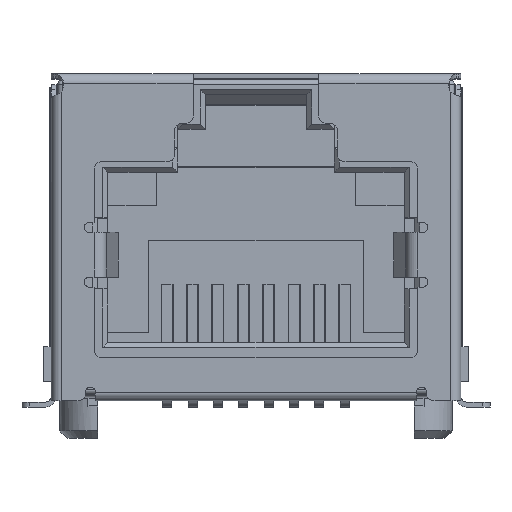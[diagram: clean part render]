
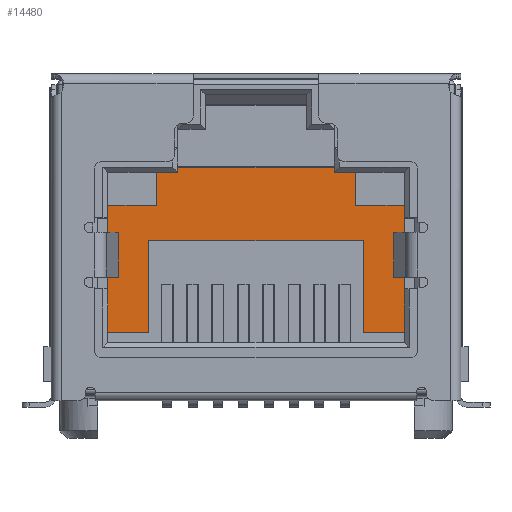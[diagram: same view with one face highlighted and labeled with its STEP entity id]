
A CAD part, top view. The second image highlights one B-rep face of the part: STEP entity #14480.
In plain terms, the highlighted planar face has unit normal (0, 0, 1).
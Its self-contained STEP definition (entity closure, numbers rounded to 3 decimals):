
#63 = ORIENTED_EDGE ( 'NONE', *, *, #17786, .T. ) ;
#538 = LINE ( 'NONE', #16832, #18644 ) ;
#540 = CARTESIAN_POINT ( 'NONE',  ( 13.93, 2.65, -12. ) ) ;
#629 = EDGE_CURVE ( 'NONE', #1205, #18476, #13843, .T. ) ;
#880 = DIRECTION ( 'NONE',  ( -1., 0., 0. ) ) ;
#1205 = VERTEX_POINT ( 'NONE', #23132 ) ;
#1334 = VECTOR ( 'NONE', #18363, 1000. ) ;
#1976 = ORIENTED_EDGE ( 'NONE', *, *, #15438, .T. ) ;
#2643 = VERTEX_POINT ( 'NONE', #22831 ) ;
#3051 = CARTESIAN_POINT ( 'NONE',  ( 3.675, 2.65, -12. ) ) ;
#3092 = LINE ( 'NONE', #10632, #17224 ) ;
#3462 = VECTOR ( 'NONE', #11119, 1000. ) ;
#3569 = CARTESIAN_POINT ( 'NONE',  ( 12.275, 2.45, -12. ) ) ;
#3611 = EDGE_CURVE ( 'NONE', #20591, #21464, #18710, .T. ) ;
#3718 = CARTESIAN_POINT ( 'NONE',  ( 2.02, 2.45, -12. ) ) ;
#4598 = CARTESIAN_POINT ( 'NONE',  ( 13.93, 9.08, -12. ) ) ;
#5008 = ORIENTED_EDGE ( 'NONE', *, *, #18022, .T. ) ;
#5014 = DIRECTION ( 'NONE',  ( -1., 0., 0. ) ) ;
#5115 = ORIENTED_EDGE ( 'NONE', *, *, #14234, .T. ) ;
#5655 = DIRECTION ( 'NONE',  ( 1., 0., 0. ) ) ;
#6001 = LINE ( 'NONE', #8613, #26694 ) ;
#6118 = VERTEX_POINT ( 'NONE', #20571 ) ;
#6464 = EDGE_CURVE ( 'NONE', #25947, #13244, #24791, .T. ) ;
#6710 = ORIENTED_EDGE ( 'NONE', *, *, #17933, .T. ) ;
#7208 = CARTESIAN_POINT ( 'NONE',  ( 2.02, 9.08, -12. ) ) ;
#7437 = EDGE_CURVE ( 'NONE', #26736, #14986, #12530, .T. ) ;
#7611 = CARTESIAN_POINT ( 'NONE',  ( 4.825, 9.08, -12. ) ) ;
#7622 = DIRECTION ( 'NONE',  ( 0., -1., 0. ) ) ;
#7928 = ORIENTED_EDGE ( 'NONE', *, *, #17822, .T. ) ;
#8017 = LINE ( 'NONE', #17445, #18201 ) ;
#8613 = CARTESIAN_POINT ( 'NONE',  ( 11.975, 7.78, -12. ) ) ;
#8751 = CARTESIAN_POINT ( 'NONE',  ( 3.675, 6.35, -12. ) ) ;
#8840 = DIRECTION ( 'NONE',  ( 0., 1., 0. ) ) ;
#9075 = LINE ( 'NONE', #23732, #3462 ) ;
#9106 = CARTESIAN_POINT ( 'NONE',  ( 2.02, 2.65, -12. ) ) ;
#9241 = CARTESIAN_POINT ( 'NONE',  ( 3.675, 2.45, -12. ) ) ;
#9522 = CARTESIAN_POINT ( 'NONE',  ( 12.275, 6.35, -12. ) ) ;
#9589 = ORIENTED_EDGE ( 'NONE', *, *, #26197, .T. ) ;
#9628 = EDGE_CURVE ( 'NONE', #2643, #21464, #10475, .T. ) ;
#9831 = VECTOR ( 'NONE', #26099, 1000. ) ;
#10428 = LINE ( 'NONE', #4598, #13393 ) ;
#10475 = LINE ( 'NONE', #19858, #9831 ) ;
#10632 = CARTESIAN_POINT ( 'NONE',  ( 2.02, 2.65, -12. ) ) ;
#10880 = EDGE_CURVE ( 'NONE', #21385, #13592, #10428, .T. ) ;
#10909 = DIRECTION ( 'NONE',  ( 0., -1., 0. ) ) ;
#11077 = CARTESIAN_POINT ( 'NONE',  ( 4.825, 9.28, -12. ) ) ;
#11104 = ORIENTED_EDGE ( 'NONE', *, *, #12902, .T. ) ;
#11119 = DIRECTION ( 'NONE',  ( 0., -1., 0. ) ) ;
#11561 = FACE_OUTER_BOUND ( 'NONE', #18744, .T. ) ;
#11934 = VECTOR ( 'NONE', #15239, 1000. ) ;
#12105 = VECTOR ( 'NONE', #25621, 1000. ) ;
#12227 = LINE ( 'NONE', #7208, #26378 ) ;
#12359 = CARTESIAN_POINT ( 'NONE',  ( 12.275, 2.65, -12. ) ) ;
#12516 = ORIENTED_EDGE ( 'NONE', *, *, #9628, .T. ) ;
#12530 = LINE ( 'NONE', #3569, #22430 ) ;
#12902 = EDGE_CURVE ( 'NONE', #20645, #2643, #9075, .T. ) ;
#12928 = LINE ( 'NONE', #12939, #23808 ) ;
#12939 = CARTESIAN_POINT ( 'NONE',  ( 11.125, 2.45, -12. ) ) ;
#13244 = VERTEX_POINT ( 'NONE', #8751 ) ;
#13393 = VECTOR ( 'NONE', #10909, 1000. ) ;
#13592 = VERTEX_POINT ( 'NONE', #16348 ) ;
#13843 = LINE ( 'NONE', #20775, #1334 ) ;
#14231 = ORIENTED_EDGE ( 'NONE', *, *, #629, .T. ) ;
#14234 = EDGE_CURVE ( 'NONE', #6118, #21433, #12227, .T. ) ;
#14480 = ADVANCED_FACE ( 'NONE', ( #11561 ), #18600, .T. ) ;
#14622 = CARTESIAN_POINT ( 'NONE',  ( 11.975, 7.78, -12. ) ) ;
#14986 = VERTEX_POINT ( 'NONE', #12359 ) ;
#15033 = EDGE_CURVE ( 'NONE', #19939, #6118, #6001, .T. ) ;
#15203 = DIRECTION ( 'NONE',  ( 0., 1., 0. ) ) ;
#15239 = DIRECTION ( 'NONE',  ( -1., 0., 0. ) ) ;
#15431 = CARTESIAN_POINT ( 'NONE',  ( 11.125, 9.08, -12. ) ) ;
#15438 = EDGE_CURVE ( 'NONE', #18476, #20645, #538, .T. ) ;
#15732 = ORIENTED_EDGE ( 'NONE', *, *, #15033, .T. ) ;
#15775 = ORIENTED_EDGE ( 'NONE', *, *, #7437, .T. ) ;
#15962 = CARTESIAN_POINT ( 'NONE',  ( 3.975, 9.08, -12. ) ) ;
#16307 = DIRECTION ( 'NONE',  ( 0., 0., 1. ) ) ;
#16348 = CARTESIAN_POINT ( 'NONE',  ( 13.93, 2.65, -12. ) ) ;
#16748 = DIRECTION ( 'NONE',  ( -1., 0., 0. ) ) ;
#16832 = CARTESIAN_POINT ( 'NONE',  ( 2.02, 9.08, -12. ) ) ;
#17097 = DIRECTION ( 'NONE',  ( 1., 0., 0. ) ) ;
#17224 = VECTOR ( 'NONE', #17097, 1000. ) ;
#17445 = CARTESIAN_POINT ( 'NONE',  ( 2.02, 6.35, -12. ) ) ;
#17756 = EDGE_CURVE ( 'NONE', #13592, #14986, #18881, .T. ) ;
#17786 = EDGE_CURVE ( 'NONE', #20591, #25947, #3092, .T. ) ;
#17822 = EDGE_CURVE ( 'NONE', #21433, #20827, #12928, .T. ) ;
#17933 = EDGE_CURVE ( 'NONE', #13244, #26736, #8017, .T. ) ;
#18022 = EDGE_CURVE ( 'NONE', #21385, #19939, #26732, .T. ) ;
#18078 = CARTESIAN_POINT ( 'NONE',  ( 2.02, 7.78, -12. ) ) ;
#18201 = VECTOR ( 'NONE', #25826, 1000. ) ;
#18363 = DIRECTION ( 'NONE',  ( 0., -1., 0. ) ) ;
#18371 = ORIENTED_EDGE ( 'NONE', *, *, #17756, .F. ) ;
#18476 = VERTEX_POINT ( 'NONE', #7611 ) ;
#18600 = PLANE ( 'NONE',  #21351 ) ;
#18644 = VECTOR ( 'NONE', #16748, 1000. ) ;
#18710 = LINE ( 'NONE', #21420, #12105 ) ;
#18743 = ORIENTED_EDGE ( 'NONE', *, *, #6464, .T. ) ;
#18744 = EDGE_LOOP ( 'NONE', ( #12516, #25174, #63, #18743, #6710, #15775, #18371, #25301, #5008, #15732, #5115, #7928, #9589, #14231, #1976, #11104 ) ) ;
#18881 = LINE ( 'NONE', #540, #11934 ) ;
#19205 = VECTOR ( 'NONE', #21920, 1000. ) ;
#19858 = CARTESIAN_POINT ( 'NONE',  ( 2.02, 7.78, -12. ) ) ;
#19939 = VERTEX_POINT ( 'NONE', #14622 ) ;
#20571 = CARTESIAN_POINT ( 'NONE',  ( 11.975, 9.08, -12. ) ) ;
#20591 = VERTEX_POINT ( 'NONE', #9106 ) ;
#20645 = VERTEX_POINT ( 'NONE', #15962 ) ;
#20775 = CARTESIAN_POINT ( 'NONE',  ( 4.825, 2.45, -12. ) ) ;
#20827 = VERTEX_POINT ( 'NONE', #20854 ) ;
#20850 = VECTOR ( 'NONE', #22329, 1000. ) ;
#20854 = CARTESIAN_POINT ( 'NONE',  ( 11.125, 9.28, -12. ) ) ;
#21351 = AXIS2_PLACEMENT_3D ( 'NONE', #3718, #16307, #5655 ) ;
#21385 = VERTEX_POINT ( 'NONE', #23109 ) ;
#21420 = CARTESIAN_POINT ( 'NONE',  ( 2.02, 2.25, -12. ) ) ;
#21433 = VERTEX_POINT ( 'NONE', #15431 ) ;
#21464 = VERTEX_POINT ( 'NONE', #23646 ) ;
#21920 = DIRECTION ( 'NONE',  ( 0., 1., 0. ) ) ;
#22329 = DIRECTION ( 'NONE',  ( -1., 0., 0. ) ) ;
#22430 = VECTOR ( 'NONE', #7622, 1000. ) ;
#22831 = CARTESIAN_POINT ( 'NONE',  ( 3.975, 7.78, -12. ) ) ;
#23109 = CARTESIAN_POINT ( 'NONE',  ( 13.93, 7.78, -12. ) ) ;
#23132 = CARTESIAN_POINT ( 'NONE',  ( 4.825, 9.28, -12. ) ) ;
#23646 = CARTESIAN_POINT ( 'NONE',  ( 2.02, 7.78, -12. ) ) ;
#23732 = CARTESIAN_POINT ( 'NONE',  ( 3.975, 9.08, -12. ) ) ;
#23808 = VECTOR ( 'NONE', #8840, 1000. ) ;
#23865 = LINE ( 'NONE', #11077, #24176 ) ;
#24176 = VECTOR ( 'NONE', #880, 1000. ) ;
#24791 = LINE ( 'NONE', #9241, #19205 ) ;
#25174 = ORIENTED_EDGE ( 'NONE', *, *, #3611, .F. ) ;
#25301 = ORIENTED_EDGE ( 'NONE', *, *, #10880, .F. ) ;
#25621 = DIRECTION ( 'NONE',  ( 0., 1., 0. ) ) ;
#25826 = DIRECTION ( 'NONE',  ( 1., 0., 0. ) ) ;
#25947 = VERTEX_POINT ( 'NONE', #3051 ) ;
#26099 = DIRECTION ( 'NONE',  ( -1., 0., 0. ) ) ;
#26197 = EDGE_CURVE ( 'NONE', #20827, #1205, #23865, .T. ) ;
#26378 = VECTOR ( 'NONE', #5014, 1000. ) ;
#26694 = VECTOR ( 'NONE', #15203, 1000. ) ;
#26732 = LINE ( 'NONE', #18078, #20850 ) ;
#26736 = VERTEX_POINT ( 'NONE', #9522 ) ;
